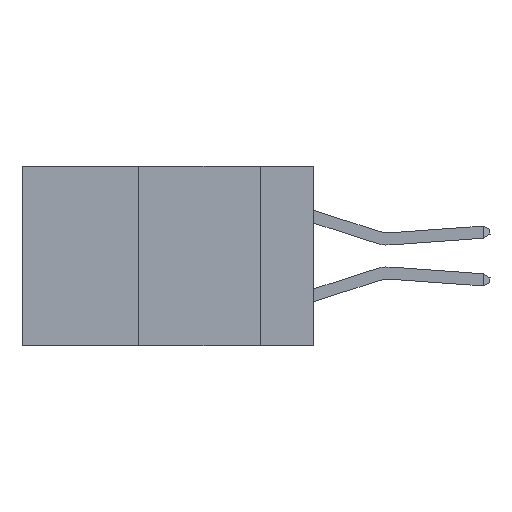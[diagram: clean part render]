
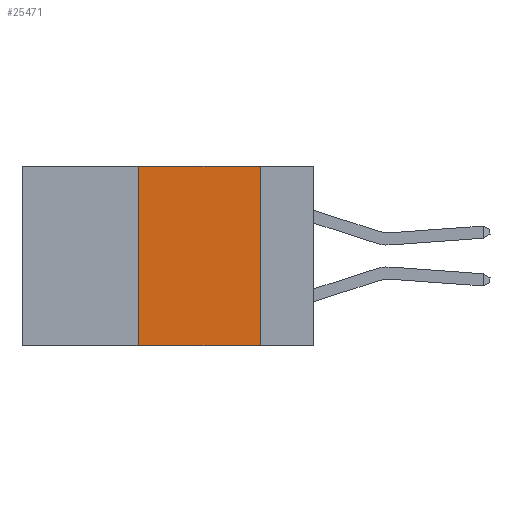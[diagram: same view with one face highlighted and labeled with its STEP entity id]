
A CAD part, left-side view. The second image highlights one B-rep face of the part: STEP entity #25471.
In plain terms, the highlighted planar face has unit normal (-1, 0, 0).
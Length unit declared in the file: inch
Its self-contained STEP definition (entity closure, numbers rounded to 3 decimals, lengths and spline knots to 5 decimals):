
#257 = VERTEX_POINT ( 'NONE', #17998 ) ;
#483 = VECTOR ( 'NONE', #19531, 39.37008 ) ;
#1103 = VERTEX_POINT ( 'NONE', #2159 ) ;
#1460 = DIRECTION ( 'NONE',  ( 0., 0., 1. ) ) ;
#2159 = CARTESIAN_POINT ( 'NONE',  ( 0., 0.11, -0.37 ) ) ;
#2999 = LINE ( 'NONE', #21664, #14896 ) ;
#3762 = ORIENTED_EDGE ( 'NONE', *, *, #4932, .F. ) ;
#4309 = VECTOR ( 'NONE', #24291, 39.37008 ) ;
#4932 = EDGE_CURVE ( 'NONE', #8221, #26613, #14267, .T. ) ;
#7288 = CARTESIAN_POINT ( 'NONE',  ( 0., 0.36, 0. ) ) ;
#8221 = VERTEX_POINT ( 'NONE', #7288 ) ;
#10532 = ORIENTED_EDGE ( 'NONE', *, *, #13104, .F. ) ;
#10851 = PLANE ( 'NONE',  #22233 ) ;
#11859 = CARTESIAN_POINT ( 'NONE',  ( 0., 0.11, 0. ) ) ;
#12093 = ORIENTED_EDGE ( 'NONE', *, *, #15426, .T. ) ;
#13104 = EDGE_CURVE ( 'NONE', #257, #8221, #2999, .T. ) ;
#13333 = CARTESIAN_POINT ( 'NONE',  ( 0., 0.6, 0. ) ) ;
#14267 = LINE ( 'NONE', #28285, #25936 ) ;
#14896 = VECTOR ( 'NONE', #1460, 39.37008 ) ;
#15426 = EDGE_CURVE ( 'NONE', #257, #1103, #20620, .T. ) ;
#15894 = DIRECTION ( 'NONE',  ( 0., 0., -1. ) ) ;
#17016 = CARTESIAN_POINT ( 'NONE',  ( 0., 0.6, -0.37 ) ) ;
#17740 = LINE ( 'NONE', #21830, #4309 ) ;
#17941 = FACE_OUTER_BOUND ( 'NONE', #23362, .T. ) ;
#17998 = CARTESIAN_POINT ( 'NONE',  ( 0., 0.36, -0.37 ) ) ;
#18147 = EDGE_CURVE ( 'NONE', #26613, #1103, #17740, .T. ) ;
#19531 = DIRECTION ( 'NONE',  ( 0., -1., 0. ) ) ;
#20620 = LINE ( 'NONE', #17016, #483 ) ;
#21664 = CARTESIAN_POINT ( 'NONE',  ( 0., 0.36, 0. ) ) ;
#21830 = CARTESIAN_POINT ( 'NONE',  ( 0., 0.11, 0. ) ) ;
#22233 = AXIS2_PLACEMENT_3D ( 'NONE', #13333, #30748, #15894 ) ;
#23362 = EDGE_LOOP ( 'NONE', ( #27735, #3762, #10532, #12093 ) ) ;
#24291 = DIRECTION ( 'NONE',  ( 0., 0., -1. ) ) ;
#25471 = ADVANCED_FACE ( 'NONE', ( #17941 ), #10851, .F. ) ;
#25936 = VECTOR ( 'NONE', #30662, 39.37008 ) ;
#26613 = VERTEX_POINT ( 'NONE', #11859 ) ;
#27735 = ORIENTED_EDGE ( 'NONE', *, *, #18147, .F. ) ;
#28285 = CARTESIAN_POINT ( 'NONE',  ( 0., 0.6, 0. ) ) ;
#30662 = DIRECTION ( 'NONE',  ( 0., -1., 0. ) ) ;
#30748 = DIRECTION ( 'NONE',  ( 1., 0., 0. ) ) ;
